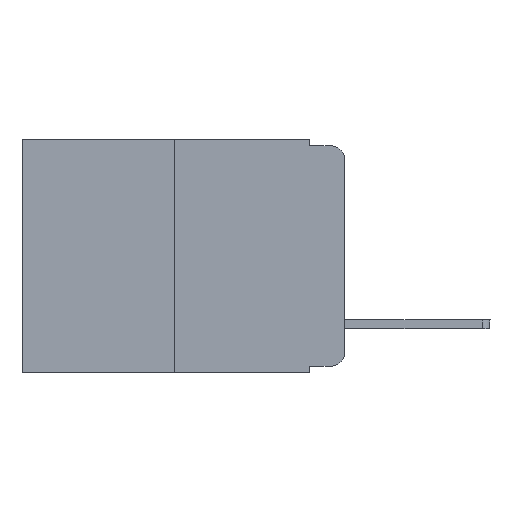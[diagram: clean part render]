
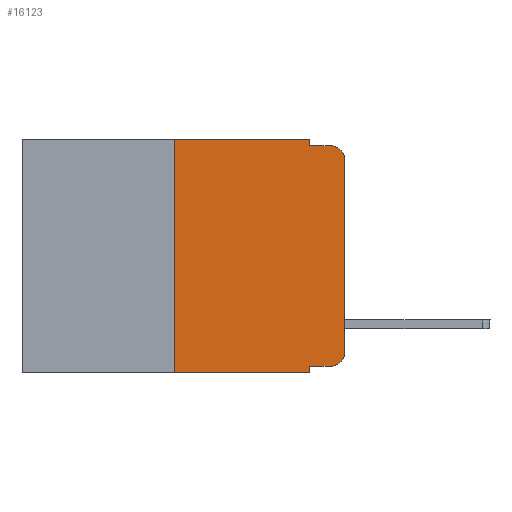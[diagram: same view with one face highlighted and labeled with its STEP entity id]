
A CAD part, left-side view. The second image highlights one B-rep face of the part: STEP entity #16123.
In plain terms, the highlighted planar face has unit normal (-1, 0, 0).
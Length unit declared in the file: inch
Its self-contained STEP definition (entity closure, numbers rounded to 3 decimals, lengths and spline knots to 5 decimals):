
#62 = DIRECTION ( 'NONE',  ( 0., 0., -1. ) ) ;
#255 = DIRECTION ( 'NONE',  ( 0., -1., 0. ) ) ;
#687 = DIRECTION ( 'NONE',  ( 0., 0., -1. ) ) ;
#1290 = EDGE_CURVE ( 'NONE', #14557, #14767, #18554, .T. ) ;
#1381 = VERTEX_POINT ( 'NONE', #17253 ) ;
#1416 = EDGE_CURVE ( 'NONE', #11379, #14557, #2236, .T. ) ;
#1502 = DIRECTION ( 'NONE',  ( -1., 0., 0. ) ) ;
#1788 = CARTESIAN_POINT ( 'NONE',  ( 0., 0.473, -0.343 ) ) ;
#2108 = PLANE ( 'NONE',  #15520 ) ;
#2231 = DIRECTION ( 'NONE',  ( 1., 0., 0. ) ) ;
#2236 = LINE ( 'NONE', #17446, #11352 ) ;
#2969 = DIRECTION ( 'NONE',  ( 0., 0., -1. ) ) ;
#3704 = CARTESIAN_POINT ( 'NONE',  ( 0., 0.473, 0. ) ) ;
#3897 = CARTESIAN_POINT ( 'NONE',  ( 0., 0.25, -0.343 ) ) ;
#4308 = VECTOR ( 'NONE', #4476, 39.37008 ) ;
#4476 = DIRECTION ( 'NONE',  ( 0., -1., 0. ) ) ;
#4605 = ORIENTED_EDGE ( 'NONE', *, *, #14157, .F. ) ;
#5139 = EDGE_CURVE ( 'NONE', #16333, #11379, #7872, .T. ) ;
#5226 = LINE ( 'NONE', #15884, #10740 ) ;
#5576 = ORIENTED_EDGE ( 'NONE', *, *, #10331, .F. ) ;
#5611 = DIRECTION ( 'NONE',  ( 0., 0., -1. ) ) ;
#5738 = VERTEX_POINT ( 'NONE', #15530 ) ;
#5853 = CARTESIAN_POINT ( 'NONE',  ( 0., 0., -0.313 ) ) ;
#6133 = CARTESIAN_POINT ( 'NONE',  ( 0., 0.02, -0.03 ) ) ;
#6328 = EDGE_CURVE ( 'NONE', #8570, #8940, #13896, .T. ) ;
#6483 = ORIENTED_EDGE ( 'NONE', *, *, #1290, .T. ) ;
#6618 = DIRECTION ( 'NONE',  ( 0., 0., -1. ) ) ;
#6628 = AXIS2_PLACEMENT_3D ( 'NONE', #6133, #1502, #2969 ) ;
#7518 = ORIENTED_EDGE ( 'NONE', *, *, #1416, .T. ) ;
#7546 = CARTESIAN_POINT ( 'NONE',  ( 0., 0.02, -0.313 ) ) ;
#7850 = CARTESIAN_POINT ( 'NONE',  ( 0., 0., -0.03 ) ) ;
#7872 = CIRCLE ( 'NONE', #17161, 0.02 ) ;
#7960 = CARTESIAN_POINT ( 'NONE',  ( 0., 0.051, -0.333 ) ) ;
#8042 = ORIENTED_EDGE ( 'NONE', *, *, #6328, .T. ) ;
#8134 = LINE ( 'NONE', #10178, #13159 ) ;
#8452 = EDGE_CURVE ( 'NONE', #1381, #16333, #18966, .T. ) ;
#8570 = VERTEX_POINT ( 'NONE', #3897 ) ;
#8786 = EDGE_CURVE ( 'NONE', #8570, #10890, #19187, .T. ) ;
#8940 = VERTEX_POINT ( 'NONE', #18987 ) ;
#9635 = DIRECTION ( 'NONE',  ( 0., -1., 0. ) ) ;
#9944 = LINE ( 'NONE', #3704, #16411 ) ;
#10178 = CARTESIAN_POINT ( 'NONE',  ( 0., 0.051, 0. ) ) ;
#10331 = EDGE_CURVE ( 'NONE', #5738, #14767, #13406, .T. ) ;
#10554 = CARTESIAN_POINT ( 'NONE',  ( 0., 0.02, -0.333 ) ) ;
#10625 = ORIENTED_EDGE ( 'NONE', *, *, #5139, .T. ) ;
#10633 = EDGE_CURVE ( 'NONE', #1381, #8940, #8134, .T. ) ;
#10740 = VECTOR ( 'NONE', #687, 39.37008 ) ;
#10890 = VERTEX_POINT ( 'NONE', #12160 ) ;
#11100 = CARTESIAN_POINT ( 'NONE',  ( 0., 0.25, 0. ) ) ;
#11352 = VECTOR ( 'NONE', #15783, 39.37008 ) ;
#11379 = VERTEX_POINT ( 'NONE', #5853 ) ;
#11885 = VERTEX_POINT ( 'NONE', #13447 ) ;
#12028 = VECTOR ( 'NONE', #18536, 39.37008 ) ;
#12160 = CARTESIAN_POINT ( 'NONE',  ( 0., 0.25, 0. ) ) ;
#13135 = DIRECTION ( 'NONE',  ( 0., -1., 0. ) ) ;
#13159 = VECTOR ( 'NONE', #5611, 39.37008 ) ;
#13406 = LINE ( 'NONE', #13650, #4308 ) ;
#13447 = CARTESIAN_POINT ( 'NONE',  ( 0., 0.051, 0. ) ) ;
#13461 = VECTOR ( 'NONE', #9635, 39.37008 ) ;
#13650 = CARTESIAN_POINT ( 'NONE',  ( 0., 0.051, -0.01 ) ) ;
#13896 = LINE ( 'NONE', #1788, #15343 ) ;
#14157 = EDGE_CURVE ( 'NONE', #10890, #11885, #9944, .T. ) ;
#14225 = ORIENTED_EDGE ( 'NONE', *, *, #18474, .F. ) ;
#14457 = CARTESIAN_POINT ( 'NONE',  ( 0., 0.02, -0.01 ) ) ;
#14557 = VERTEX_POINT ( 'NONE', #7850 ) ;
#14735 = EDGE_LOOP ( 'NONE', ( #7518, #6483, #5576, #14225, #4605, #17520, #8042, #14799, #18155, #10625 ) ) ;
#14767 = VERTEX_POINT ( 'NONE', #14457 ) ;
#14799 = ORIENTED_EDGE ( 'NONE', *, *, #10633, .F. ) ;
#15343 = VECTOR ( 'NONE', #255, 39.37008 ) ;
#15520 = AXIS2_PLACEMENT_3D ( 'NONE', #16034, #2231, #6618 ) ;
#15530 = CARTESIAN_POINT ( 'NONE',  ( 0., 0.051, -0.01 ) ) ;
#15783 = DIRECTION ( 'NONE',  ( 0., 0., 1. ) ) ;
#15884 = CARTESIAN_POINT ( 'NONE',  ( 0., 0.051, 0. ) ) ;
#16034 = CARTESIAN_POINT ( 'NONE',  ( 0., 0.473, 0. ) ) ;
#16123 = ADVANCED_FACE ( 'NONE', ( #17488 ), #2108, .F. ) ;
#16333 = VERTEX_POINT ( 'NONE', #10554 ) ;
#16411 = VECTOR ( 'NONE', #13135, 39.37008 ) ;
#17161 = AXIS2_PLACEMENT_3D ( 'NONE', #7546, #18256, #62 ) ;
#17253 = CARTESIAN_POINT ( 'NONE',  ( 0., 0.051, -0.333 ) ) ;
#17446 = CARTESIAN_POINT ( 'NONE',  ( 0., 0., 0. ) ) ;
#17488 = FACE_OUTER_BOUND ( 'NONE', #14735, .T. ) ;
#17520 = ORIENTED_EDGE ( 'NONE', *, *, #8786, .F. ) ;
#18155 = ORIENTED_EDGE ( 'NONE', *, *, #8452, .T. ) ;
#18256 = DIRECTION ( 'NONE',  ( -1., 0., 0. ) ) ;
#18474 = EDGE_CURVE ( 'NONE', #11885, #5738, #5226, .T. ) ;
#18536 = DIRECTION ( 'NONE',  ( 0., 0., 1. ) ) ;
#18554 = CIRCLE ( 'NONE', #6628, 0.02 ) ;
#18966 = LINE ( 'NONE', #7960, #13461 ) ;
#18987 = CARTESIAN_POINT ( 'NONE',  ( 0., 0.051, -0.343 ) ) ;
#19187 = LINE ( 'NONE', #11100, #12028 ) ;
